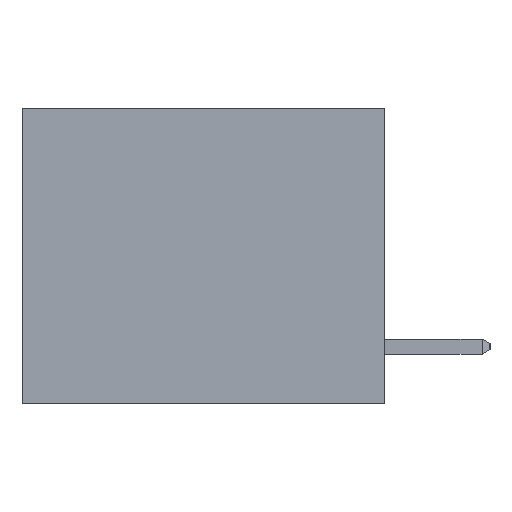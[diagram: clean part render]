
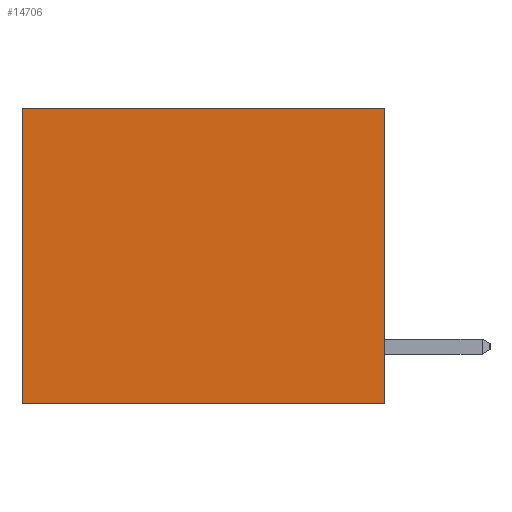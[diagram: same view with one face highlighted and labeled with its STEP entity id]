
A CAD part, left-side view. The second image highlights one B-rep face of the part: STEP entity #14706.
In plain terms, the highlighted planar face has unit normal (-1, 0, 0).
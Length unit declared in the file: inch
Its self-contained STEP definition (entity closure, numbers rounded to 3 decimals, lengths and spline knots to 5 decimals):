
#997 = ORIENTED_EDGE ( 'NONE', *, *, #15137, .F. ) ;
#1501 = CARTESIAN_POINT ( 'NONE',  ( 0.3165, 0.6, -0.49 ) ) ;
#2062 = DIRECTION ( 'NONE',  ( 0., 0., -1. ) ) ;
#2943 = VERTEX_POINT ( 'NONE', #10449 ) ;
#3120 = VECTOR ( 'NONE', #2062, 39.37008 ) ;
#3241 = CARTESIAN_POINT ( 'NONE',  ( 0.3165, 0.6, 0. ) ) ;
#3242 = ORIENTED_EDGE ( 'NONE', *, *, #14499, .T. ) ;
#3563 = CARTESIAN_POINT ( 'NONE',  ( 0.3165, 0.6, -0.49 ) ) ;
#4102 = AXIS2_PLACEMENT_3D ( 'NONE', #18021, #4428, #12260 ) ;
#4428 = DIRECTION ( 'NONE',  ( 1., 0., 0. ) ) ;
#4562 = PLANE ( 'NONE',  #4102 ) ;
#6008 = LINE ( 'NONE', #7915, #14751 ) ;
#6851 = CARTESIAN_POINT ( 'NONE',  ( 0.3165, 0., 0. ) ) ;
#7901 = LINE ( 'NONE', #12739, #18577 ) ;
#7915 = CARTESIAN_POINT ( 'NONE',  ( 0.3165, 0., -0.49 ) ) ;
#8174 = CARTESIAN_POINT ( 'NONE',  ( 0.3165, 0., 0. ) ) ;
#8378 = DIRECTION ( 'NONE',  ( 0., 1., 0. ) ) ;
#9040 = EDGE_CURVE ( 'NONE', #2943, #9526, #6008, .T. ) ;
#9289 = VERTEX_POINT ( 'NONE', #6851 ) ;
#9310 = DIRECTION ( 'NONE',  ( 0., 1., 0. ) ) ;
#9509 = ORIENTED_EDGE ( 'NONE', *, *, #11712, .T. ) ;
#9526 = VERTEX_POINT ( 'NONE', #1501 ) ;
#10449 = CARTESIAN_POINT ( 'NONE',  ( 0.3165, 0., -0.49 ) ) ;
#10854 = VECTOR ( 'NONE', #8378, 39.37008 ) ;
#11712 = EDGE_CURVE ( 'NONE', #9289, #14388, #18934, .T. ) ;
#11751 = ORIENTED_EDGE ( 'NONE', *, *, #9040, .F. ) ;
#12260 = DIRECTION ( 'NONE',  ( 0., 0., -1. ) ) ;
#12739 = CARTESIAN_POINT ( 'NONE',  ( 0.3165, 0., -0.49 ) ) ;
#14388 = VERTEX_POINT ( 'NONE', #3241 ) ;
#14499 = EDGE_CURVE ( 'NONE', #14388, #9526, #17217, .T. ) ;
#14706 = ADVANCED_FACE ( 'NONE', ( #15011 ), #4562, .F. ) ;
#14751 = VECTOR ( 'NONE', #9310, 39.37008 ) ;
#15011 = FACE_OUTER_BOUND ( 'NONE', #16304, .T. ) ;
#15137 = EDGE_CURVE ( 'NONE', #9289, #2943, #7901, .T. ) ;
#16304 = EDGE_LOOP ( 'NONE', ( #3242, #11751, #997, #9509 ) ) ;
#17171 = DIRECTION ( 'NONE',  ( 0., 0., -1. ) ) ;
#17217 = LINE ( 'NONE', #3563, #3120 ) ;
#18021 = CARTESIAN_POINT ( 'NONE',  ( 0.3165, 0., -0.49 ) ) ;
#18577 = VECTOR ( 'NONE', #17171, 39.37008 ) ;
#18934 = LINE ( 'NONE', #8174, #10854 ) ;
